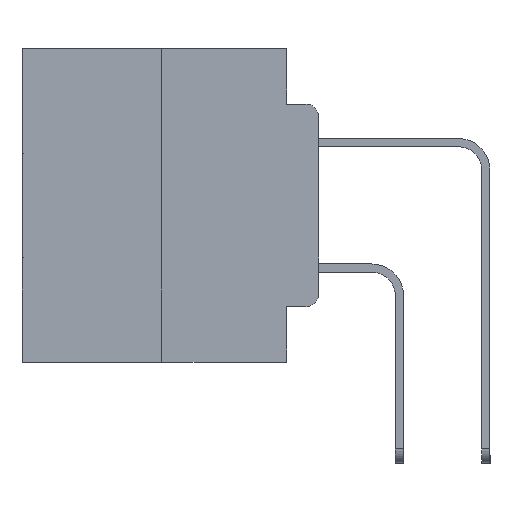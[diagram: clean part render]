
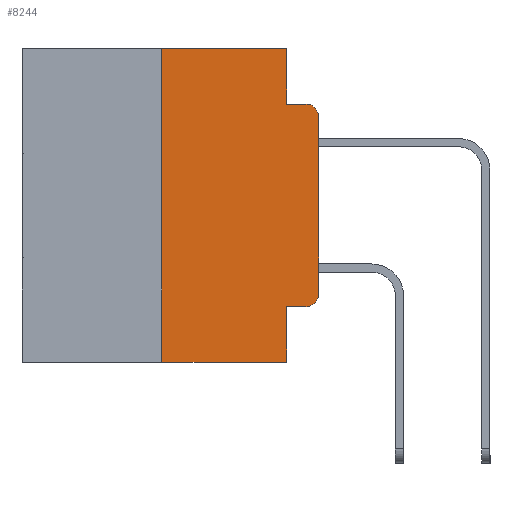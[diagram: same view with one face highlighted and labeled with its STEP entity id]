
A CAD part, left-side view. The second image highlights one B-rep face of the part: STEP entity #8244.
In plain terms, the highlighted planar face has unit normal (-1, 0, 0).
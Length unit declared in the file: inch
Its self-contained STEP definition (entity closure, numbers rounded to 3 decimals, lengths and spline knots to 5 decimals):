
#255 = ORIENTED_EDGE ( 'NONE', *, *, #8085, .F. ) ;
#284 = ORIENTED_EDGE ( 'NONE', *, *, #3707, .T. ) ;
#873 = DIRECTION ( 'NONE',  ( -1., 0., 0. ) ) ;
#1011 = ORIENTED_EDGE ( 'NONE', *, *, #6480, .F. ) ;
#1150 = VERTEX_POINT ( 'NONE', #1729 ) ;
#1225 = AXIS2_PLACEMENT_3D ( 'NONE', #14923, #873, #17215 ) ;
#1303 = EDGE_LOOP ( 'NONE', ( #26408, #17429, #5790, #27476, #26743, #255, #284, #1011, #2414, #5593 ) ) ;
#1583 = CARTESIAN_POINT ( 'NONE',  ( 0., 0.051, 0. ) ) ;
#1729 = CARTESIAN_POINT ( 'NONE',  ( 0., 0.051, -0.4115 ) ) ;
#2187 = CIRCLE ( 'NONE', #19823, 0.02 ) ;
#2414 = ORIENTED_EDGE ( 'NONE', *, *, #4911, .T. ) ;
#3322 = EDGE_CURVE ( 'NONE', #11419, #23275, #2187, .T. ) ;
#3707 = EDGE_CURVE ( 'NONE', #5959, #14165, #12349, .T. ) ;
#3714 = VECTOR ( 'NONE', #24521, 39.37008 ) ;
#3926 = DIRECTION ( 'NONE',  ( -1., 0., 0. ) ) ;
#4676 = DIRECTION ( 'NONE',  ( 0., 0., -1. ) ) ;
#4892 = LINE ( 'NONE', #8087, #28363 ) ;
#4911 = EDGE_CURVE ( 'NONE', #1150, #11419, #4892, .T. ) ;
#5593 = ORIENTED_EDGE ( 'NONE', *, *, #3322, .T. ) ;
#5615 = VERTEX_POINT ( 'NONE', #28583 ) ;
#5790 = ORIENTED_EDGE ( 'NONE', *, *, #12806, .F. ) ;
#5959 = VERTEX_POINT ( 'NONE', #25370 ) ;
#6480 = EDGE_CURVE ( 'NONE', #1150, #14165, #7802, .T. ) ;
#6845 = DIRECTION ( 'NONE',  ( 0., -1., 0. ) ) ;
#7014 = CARTESIAN_POINT ( 'NONE',  ( 0., 0.02, -0.3915 ) ) ;
#7150 = DIRECTION ( 'NONE',  ( 0., -1., 0. ) ) ;
#7275 = DIRECTION ( 'NONE',  ( 0., 0., -1. ) ) ;
#7360 = LINE ( 'NONE', #24888, #18908 ) ;
#7802 = LINE ( 'NONE', #20997, #14014 ) ;
#8085 = EDGE_CURVE ( 'NONE', #5959, #18181, #14272, .T. ) ;
#8087 = CARTESIAN_POINT ( 'NONE',  ( 0., 0.051, -0.4115 ) ) ;
#8244 = ADVANCED_FACE ( 'NONE', ( #9173 ), #29609, .F. ) ;
#8564 = CIRCLE ( 'NONE', #1225, 0.02 ) ;
#9173 = FACE_OUTER_BOUND ( 'NONE', #1303, .T. ) ;
#10029 = LINE ( 'NONE', #11191, #3714 ) ;
#10462 = DIRECTION ( 'NONE',  ( 0., -1., 0. ) ) ;
#10474 = VERTEX_POINT ( 'NONE', #19637 ) ;
#10766 = AXIS2_PLACEMENT_3D ( 'NONE', #16301, #18570, #4676 ) ;
#11191 = CARTESIAN_POINT ( 'NONE',  ( 0., 0.473, 0. ) ) ;
#11258 = EDGE_CURVE ( 'NONE', #10474, #5615, #12128, .T. ) ;
#11419 = VERTEX_POINT ( 'NONE', #16270 ) ;
#11616 = DIRECTION ( 'NONE',  ( 0., 0., -1. ) ) ;
#11890 = CARTESIAN_POINT ( 'NONE',  ( 0., 0.051, -0.0885 ) ) ;
#12128 = LINE ( 'NONE', #1583, #17487 ) ;
#12325 = CARTESIAN_POINT ( 'NONE',  ( 0., 0.25, 0. ) ) ;
#12349 = LINE ( 'NONE', #27550, #18397 ) ;
#12806 = EDGE_CURVE ( 'NONE', #5615, #23892, #25698, .T. ) ;
#13429 = DIRECTION ( 'NONE',  ( 0., 0., 1. ) ) ;
#13552 = CARTESIAN_POINT ( 'NONE',  ( 0., 0., -0.3915 ) ) ;
#14014 = VECTOR ( 'NONE', #7275, 39.37008 ) ;
#14165 = VERTEX_POINT ( 'NONE', #26281 ) ;
#14272 = LINE ( 'NONE', #29042, #19584 ) ;
#14923 = CARTESIAN_POINT ( 'NONE',  ( 0., 0.02, -0.1085 ) ) ;
#15595 = DIRECTION ( 'NONE',  ( 0., 0., -1. ) ) ;
#15618 = CARTESIAN_POINT ( 'NONE',  ( 0., 0., -0.1085 ) ) ;
#15867 = EDGE_CURVE ( 'NONE', #16073, #23892, #8564, .T. ) ;
#16073 = VERTEX_POINT ( 'NONE', #15618 ) ;
#16270 = CARTESIAN_POINT ( 'NONE',  ( 0., 0.02, -0.4115 ) ) ;
#16301 = CARTESIAN_POINT ( 'NONE',  ( 0., 0.473, 0. ) ) ;
#16644 = EDGE_CURVE ( 'NONE', #18181, #10474, #10029, .T. ) ;
#17215 = DIRECTION ( 'NONE',  ( 0., 0., -1. ) ) ;
#17388 = EDGE_CURVE ( 'NONE', #23275, #16073, #7360, .T. ) ;
#17429 = ORIENTED_EDGE ( 'NONE', *, *, #15867, .T. ) ;
#17487 = VECTOR ( 'NONE', #15595, 39.37008 ) ;
#18181 = VERTEX_POINT ( 'NONE', #12325 ) ;
#18397 = VECTOR ( 'NONE', #6845, 39.37008 ) ;
#18443 = VECTOR ( 'NONE', #7150, 39.37008 ) ;
#18570 = DIRECTION ( 'NONE',  ( 1., 0., 0. ) ) ;
#18908 = VECTOR ( 'NONE', #27127, 39.37008 ) ;
#19584 = VECTOR ( 'NONE', #13429, 39.37008 ) ;
#19637 = CARTESIAN_POINT ( 'NONE',  ( 0., 0.051, 0. ) ) ;
#19823 = AXIS2_PLACEMENT_3D ( 'NONE', #7014, #3926, #11616 ) ;
#20997 = CARTESIAN_POINT ( 'NONE',  ( 0., 0.051, 0. ) ) ;
#23275 = VERTEX_POINT ( 'NONE', #13552 ) ;
#23892 = VERTEX_POINT ( 'NONE', #24636 ) ;
#24521 = DIRECTION ( 'NONE',  ( 0., -1., 0. ) ) ;
#24636 = CARTESIAN_POINT ( 'NONE',  ( 0., 0.02, -0.0885 ) ) ;
#24888 = CARTESIAN_POINT ( 'NONE',  ( 0., 0., 0. ) ) ;
#25370 = CARTESIAN_POINT ( 'NONE',  ( 0., 0.25, -0.5 ) ) ;
#25698 = LINE ( 'NONE', #11890, #18443 ) ;
#26281 = CARTESIAN_POINT ( 'NONE',  ( 0., 0.051, -0.5 ) ) ;
#26408 = ORIENTED_EDGE ( 'NONE', *, *, #17388, .T. ) ;
#26743 = ORIENTED_EDGE ( 'NONE', *, *, #16644, .F. ) ;
#27127 = DIRECTION ( 'NONE',  ( 0., 0., 1. ) ) ;
#27476 = ORIENTED_EDGE ( 'NONE', *, *, #11258, .F. ) ;
#27550 = CARTESIAN_POINT ( 'NONE',  ( 0., 0.473, -0.5 ) ) ;
#28363 = VECTOR ( 'NONE', #10462, 39.37008 ) ;
#28583 = CARTESIAN_POINT ( 'NONE',  ( 0., 0.051, -0.0885 ) ) ;
#29042 = CARTESIAN_POINT ( 'NONE',  ( 0., 0.25, 0. ) ) ;
#29609 = PLANE ( 'NONE',  #10766 ) ;
